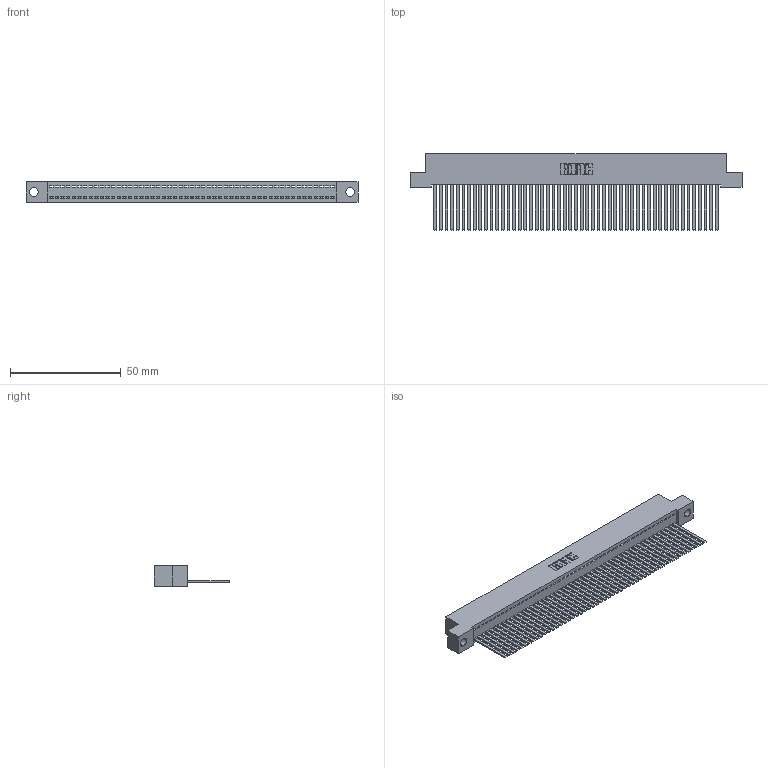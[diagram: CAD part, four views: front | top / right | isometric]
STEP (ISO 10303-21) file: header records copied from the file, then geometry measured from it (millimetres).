
FILE_DESCRIPTION (( 'STEP AP203' ), '1' );
FILE_NAME ('392-051-544-104.STEP', '2019-10-08T12:05:19', ( '' ), ( '' ), 'SwSTEP 2.0', 'SolidWorks 2016', '' );
FILE_SCHEMA (( 'CONFIG_CONTROL_DESIGN' ));
Length unit declared in the file: inch
Products named in the file (3): 342 Part_.156 TH; 345-292-001_345-293-144; 392-051-544-104
Assembly tree (52 placements, depth 2):
  392-051-544-104
    342 Part_.156 TH
    345-292-001_345-293-144  x51
Bounding box: 149.86 x 34.3 x 9.4 mm (x, y, z)
Volume: 13676.5 mm3; surface area: 21751.2 mm2
Topology: 52 solids, 52 shells, 2762 faces, 8357 edges, 5502 vertices
Faces by surface type: plane 2004, cylinder 758
Entity records: 29701 total; most frequent: CARTESIAN_POINT 5127, ORIENTED_EDGE 5114, DIRECTION 4303, EDGE_CURVE 2557, VECTOR 2433, LINE 2433, VERTEX_POINT 1702, AXIS2_PLACEMENT_3D 935
